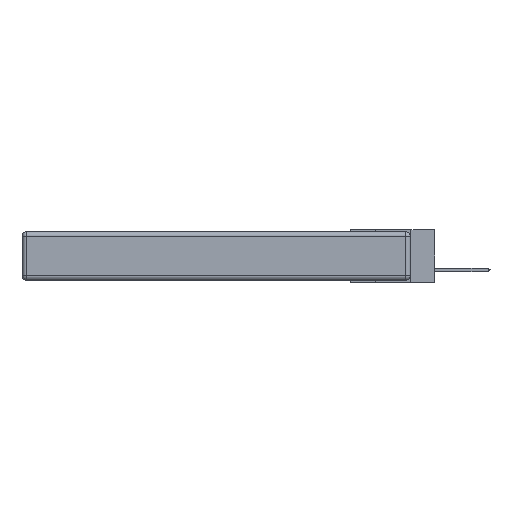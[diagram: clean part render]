
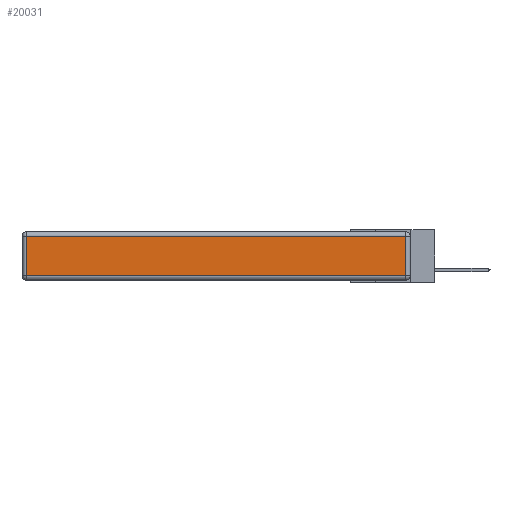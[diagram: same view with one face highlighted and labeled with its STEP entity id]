
A CAD part, left-side view. The second image highlights one B-rep face of the part: STEP entity #20031.
In plain terms, the highlighted planar face has unit normal (-1, 0, 0).
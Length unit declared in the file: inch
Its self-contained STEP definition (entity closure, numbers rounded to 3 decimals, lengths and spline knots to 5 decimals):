
#1927 = DIRECTION ( 'NONE',  ( 0., 1., 0. ) ) ;
#3901 = VERTEX_POINT ( 'NONE', #15973 ) ;
#5771 = ORIENTED_EDGE ( 'NONE', *, *, #19385, .T. ) ;
#5850 = DIRECTION ( 'NONE',  ( -1., 0., 0. ) ) ;
#6040 = DIRECTION ( 'NONE',  ( 0., 0., -1. ) ) ;
#6700 = LINE ( 'NONE', #6752, #10694 ) ;
#6752 = CARTESIAN_POINT ( 'NONE',  ( 0., 0.03, -0.343 ) ) ;
#7086 = AXIS2_PLACEMENT_3D ( 'NONE', #9667, #5850, #13754 ) ;
#7488 = VECTOR ( 'NONE', #21863, 39.37008 ) ;
#9667 = CARTESIAN_POINT ( 'NONE',  ( 0., 0., -0.343 ) ) ;
#10202 = VERTEX_POINT ( 'NONE', #13025 ) ;
#10694 = VECTOR ( 'NONE', #16850, 39.37008 ) ;
#11556 = ORIENTED_EDGE ( 'NONE', *, *, #20944, .T. ) ;
#11715 = CARTESIAN_POINT ( 'NONE',  ( 0., 2.75, -0.03 ) ) ;
#12032 = VERTEX_POINT ( 'NONE', #12131 ) ;
#12035 = CARTESIAN_POINT ( 'NONE',  ( 0., 0., -0.313 ) ) ;
#12131 = CARTESIAN_POINT ( 'NONE',  ( 0., 0.03, -0.313 ) ) ;
#13025 = CARTESIAN_POINT ( 'NONE',  ( 0., 0.03, -0.03 ) ) ;
#13754 = DIRECTION ( 'NONE',  ( 0., 0., 1. ) ) ;
#13920 = PLANE ( 'NONE',  #7086 ) ;
#14165 = VECTOR ( 'NONE', #6040, 39.37008 ) ;
#15199 = LINE ( 'NONE', #12035, #7488 ) ;
#15973 = CARTESIAN_POINT ( 'NONE',  ( 0., 2.72, -0.313 ) ) ;
#16008 = VECTOR ( 'NONE', #1927, 39.37008 ) ;
#16850 = DIRECTION ( 'NONE',  ( 0., 0., 1. ) ) ;
#17442 = FACE_OUTER_BOUND ( 'NONE', #23962, .T. ) ;
#17860 = CARTESIAN_POINT ( 'NONE',  ( 0., 2.72, -0.343 ) ) ;
#18148 = EDGE_CURVE ( 'NONE', #10202, #18167, #20061, .T. ) ;
#18167 = VERTEX_POINT ( 'NONE', #21679 ) ;
#19191 = ORIENTED_EDGE ( 'NONE', *, *, #18148, .T. ) ;
#19385 = EDGE_CURVE ( 'NONE', #18167, #3901, #21668, .T. ) ;
#20031 = ADVANCED_FACE ( 'NONE', ( #17442 ), #13920, .T. ) ;
#20061 = LINE ( 'NONE', #11715, #16008 ) ;
#20063 = ORIENTED_EDGE ( 'NONE', *, *, #22401, .T. ) ;
#20944 = EDGE_CURVE ( 'NONE', #3901, #12032, #15199, .T. ) ;
#21668 = LINE ( 'NONE', #17860, #14165 ) ;
#21679 = CARTESIAN_POINT ( 'NONE',  ( 0., 2.72, -0.03 ) ) ;
#21863 = DIRECTION ( 'NONE',  ( 0., -1., 0. ) ) ;
#22401 = EDGE_CURVE ( 'NONE', #12032, #10202, #6700, .T. ) ;
#23962 = EDGE_LOOP ( 'NONE', ( #11556, #20063, #19191, #5771 ) ) ;
